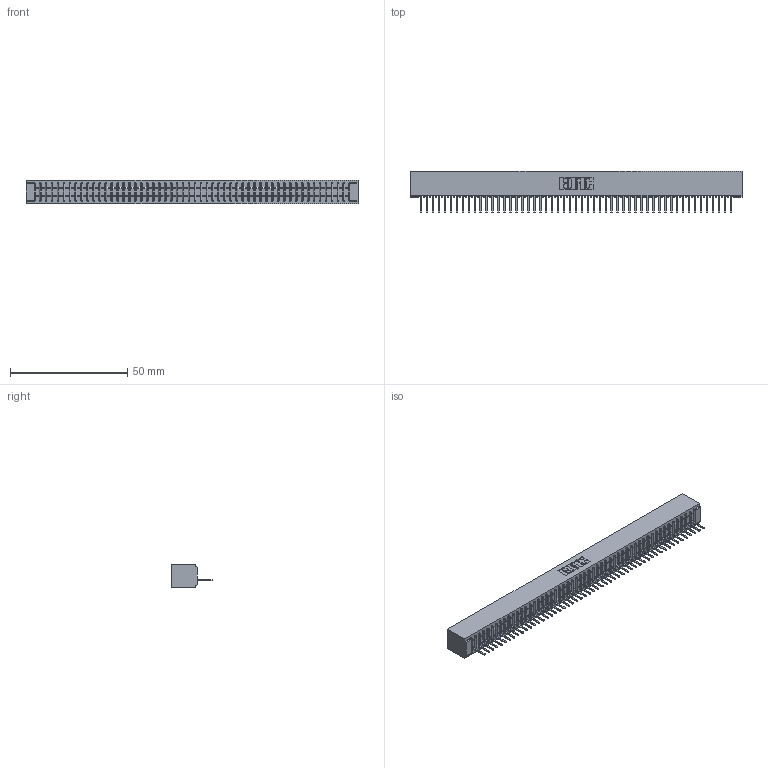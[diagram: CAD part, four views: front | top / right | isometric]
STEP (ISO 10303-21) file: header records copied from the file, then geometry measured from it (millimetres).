
FILE_DESCRIPTION (( 'STEP AP203' ), '1' );
FILE_NAME ('391-053-521-101.STEP', '2018-08-09T06:32:31', ( '' ), ( '' ), 'SwSTEP 2.0', 'SolidWorks 2016', '' );
FILE_SCHEMA (( 'CONFIG_CONTROL_DESIGN' ));
Length unit declared in the file: inch
Products named in the file (3): 341 Part_No Mounting Lugs; 341-292-001_341-292-121; 391-053-521-101
Assembly tree (54 placements, depth 2):
  391-053-521-101
    341 Part_No Mounting Lugs
    341-292-001_341-292-121  x53
Bounding box: 141.6 x 17.7 x 10.16 mm (x, y, z)
Volume: 10363.3 mm3; surface area: 16999.9 mm2
Topology: 54 solids, 54 shells, 4454 faces, 12853 edges, 8246 vertices
Faces by surface type: plane 2767, cylinder 1475, sphere 108, torus 104
Entity records: 60702 total; most frequent: CARTESIAN_POINT 10318, ORIENTED_EDGE 10306, DIRECTION 9949, EDGE_CURVE 5153, LINE 4179, VECTOR 4179, VERTEX_POINT 3254, AXIS2_PLACEMENT_3D 2885
